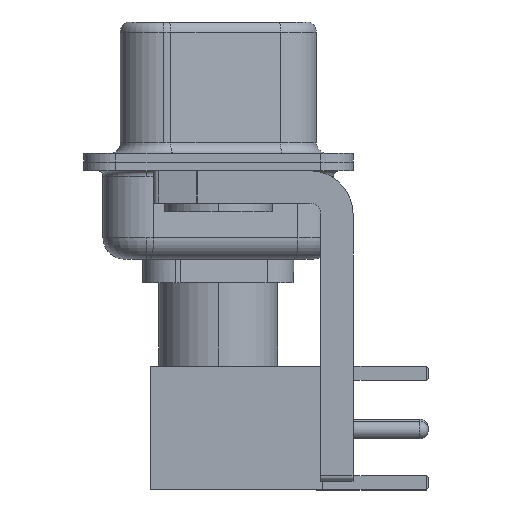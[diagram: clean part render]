
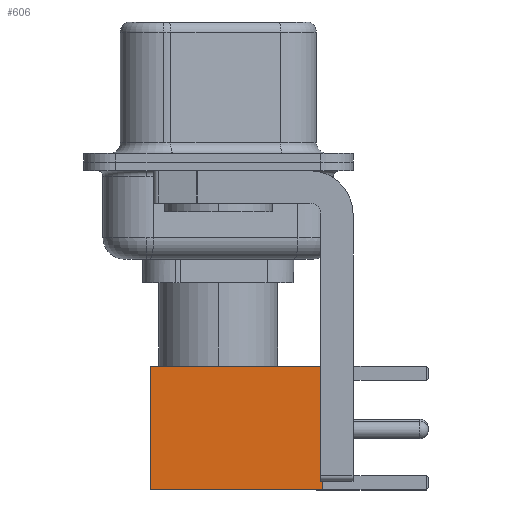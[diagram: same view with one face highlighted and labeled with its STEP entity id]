
A CAD part, left-side view. The second image highlights one B-rep face of the part: STEP entity #606.
In plain terms, the highlighted face is planar.
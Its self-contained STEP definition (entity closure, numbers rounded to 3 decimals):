
#210 = CARTESIAN_POINT ( 'NONE',  ( -2.875, 2.875, 0. ) ) ;
#293 = DIRECTION ( 'NONE',  ( -1., 0., 0. ) ) ;
#606 = ADVANCED_FACE ( 'NONE', ( #6641 ), #4879, .T. ) ;
#994 = DIRECTION ( 'NONE',  ( 0., 0., -1. ) ) ;
#1376 = EDGE_LOOP ( 'NONE', ( #11144, #7741, #10343, #11411 ) ) ;
#2098 = DIRECTION ( 'NONE',  ( 0., 0., 1. ) ) ;
#2728 = LINE ( 'NONE', #8988, #12298 ) ;
#4626 = VERTEX_POINT ( 'NONE', #8721 ) ;
#4879 = PLANE ( 'NONE',  #18021 ) ;
#6446 = VERTEX_POINT ( 'NONE', #14522 ) ;
#6641 = FACE_OUTER_BOUND ( 'NONE', #1376, .T. ) ;
#6733 = DIRECTION ( 'NONE',  ( 0., 1., 0. ) ) ;
#7673 = EDGE_CURVE ( 'NONE', #12775, #6446, #13232, .T. ) ;
#7741 = ORIENTED_EDGE ( 'NONE', *, *, #19707, .T. ) ;
#8224 = VECTOR ( 'NONE', #20268, 1000. ) ;
#8721 = CARTESIAN_POINT ( 'NONE',  ( 2.875, 2.875, 0. ) ) ;
#8988 = CARTESIAN_POINT ( 'NONE',  ( 2.875, 2.875, 0. ) ) ;
#9541 = VECTOR ( 'NONE', #293, 1000. ) ;
#10343 = ORIENTED_EDGE ( 'NONE', *, *, #19899, .F. ) ;
#11144 = ORIENTED_EDGE ( 'NONE', *, *, #13531, .T. ) ;
#11411 = ORIENTED_EDGE ( 'NONE', *, *, #7673, .F. ) ;
#11816 = CARTESIAN_POINT ( 'NONE',  ( 0., 2.875, 8. ) ) ;
#11862 = LINE ( 'NONE', #14003, #8224 ) ;
#12114 = VECTOR ( 'NONE', #18081, 1000. ) ;
#12298 = VECTOR ( 'NONE', #994, 1000. ) ;
#12775 = VERTEX_POINT ( 'NONE', #13199 ) ;
#13199 = CARTESIAN_POINT ( 'NONE',  ( 2.875, 2.875, 8. ) ) ;
#13232 = LINE ( 'NONE', #11816, #12114 ) ;
#13531 = EDGE_CURVE ( 'NONE', #12775, #4626, #2728, .T. ) ;
#14003 = CARTESIAN_POINT ( 'NONE',  ( -2.875, 2.875, 0. ) ) ;
#14318 = CARTESIAN_POINT ( 'NONE',  ( 0., 2.875, 0. ) ) ;
#14522 = CARTESIAN_POINT ( 'NONE',  ( -2.875, 2.875, 8. ) ) ;
#15870 = LINE ( 'NONE', #14318, #9541 ) ;
#17593 = CARTESIAN_POINT ( 'NONE',  ( 2.875, 2.875, 0. ) ) ;
#18021 = AXIS2_PLACEMENT_3D ( 'NONE', #17593, #6733, #2098 ) ;
#18081 = DIRECTION ( 'NONE',  ( -1., 0., 0. ) ) ;
#19074 = VERTEX_POINT ( 'NONE', #210 ) ;
#19707 = EDGE_CURVE ( 'NONE', #4626, #19074, #15870, .T. ) ;
#19899 = EDGE_CURVE ( 'NONE', #6446, #19074, #11862, .T. ) ;
#20268 = DIRECTION ( 'NONE',  ( 0., 0., -1. ) ) ;
